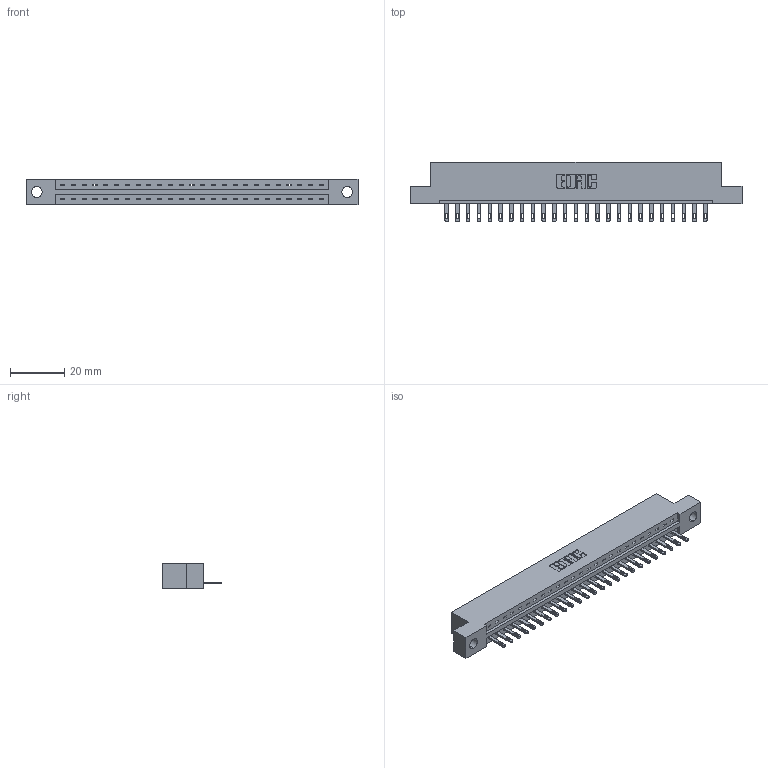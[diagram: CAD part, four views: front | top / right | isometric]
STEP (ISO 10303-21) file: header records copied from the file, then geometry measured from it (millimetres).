
FILE_DESCRIPTION (( 'STEP AP203' ), '1' );
FILE_NAME ('887-025-500-104.STEP', '2020-09-20T19:19:25', ( '' ), ( '' ), 'SwSTEP 2.0', 'SolidWorks 2020', '' );
FILE_SCHEMA (( 'CONFIG_CONTROL_DESIGN' ));
Length unit declared in the file: inch
Products named in the file (3): 887-025-500-104; 837 Part_Flush Mounting Lugs - 0.156 Dia-TH; 345-292-001_345-293-100
Assembly tree (26 placements, depth 2):
  887-025-500-104
    837 Part_Flush Mounting Lugs - 0.156 Dia-TH
    345-292-001_345-293-100  x25
Bounding box: 122.07 x 21.85 x 9.4 mm (x, y, z)
Volume: 12402.3 mm3; surface area: 12575.2 mm2
Topology: 26 solids, 26 shells, 1564 faces, 4811 edges, 3206 vertices
Faces by surface type: plane 1070, cylinder 494
Entity records: 20715 total; most frequent: CARTESIAN_POINT 3613, ORIENTED_EDGE 3574, DIRECTION 3077, EDGE_CURVE 1787, LINE 1655, VECTOR 1655, VERTEX_POINT 1190, AXIS2_PLACEMENT_3D 711
